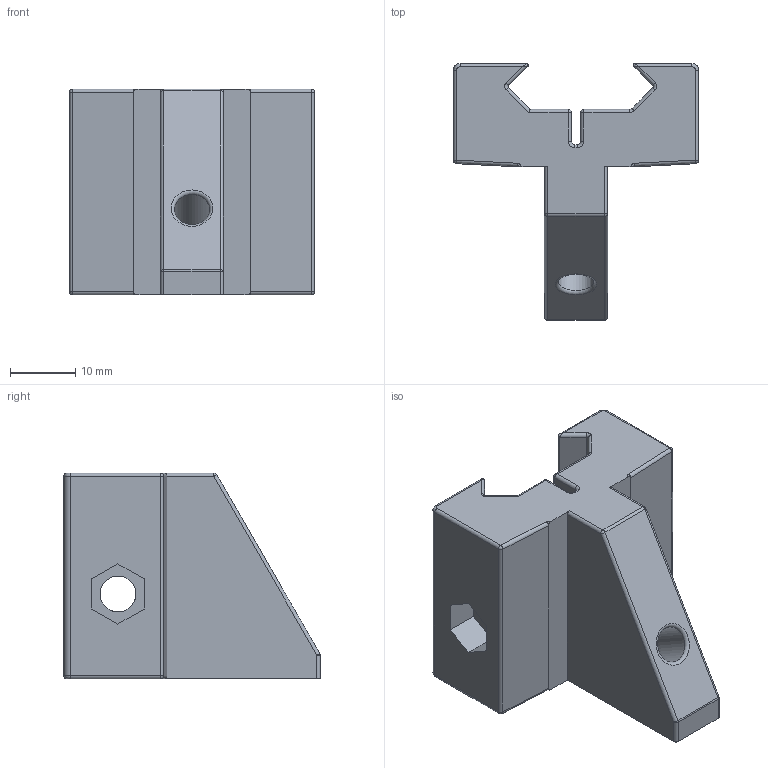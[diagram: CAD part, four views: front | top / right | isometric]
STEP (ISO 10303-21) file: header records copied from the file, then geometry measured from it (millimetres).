
FILE_DESCRIPTION(/* description */ (''),/* implementation_level */ '2;1');
FILE_NAME(/* name */ 'foregrip-adapter-picc-freeman1337.step',/* time_stamp */ '2021-04-05T12:08:16-07:00',/* author */ (''),/* organization */ (''),/* preprocessor_version */ 'ST-DEVELOPER v18.1',/* originating_system */ 'Autodesk Translation Framework v9.10.0.1330',/* authorisation */ '');
FILE_SCHEMA (('AUTOMOTIVE_DESIGN { 1 0 10303 214 3 1 1 }'));
Length unit declared in the file: millimetre
Products named in the file (1): adapter-picc
Bounding box: 37.5 x 39.25 x 31.5 mm (x, y, z)
Volume: 17381.7 mm3; surface area: 7129.6 mm2
Topology: 1 solids, 1 shells, 130 faces, 307 edges, 172 vertices
Faces by surface type: cylinder 58, plane 34, torus 14, bspline 12, sphere 12
Full cylindrical faces by diameter (mm): 5.41 x1, 5.5 x2, 9.75 x1
Entity records: 3910 total; most frequent: CARTESIAN_POINT 894, DIRECTION 677, ORIENTED_EDGE 598, EDGE_CURVE 299, AXIS2_PLACEMENT_3D 265, VERTEX_POINT 172, LINE 147, VECTOR 147
